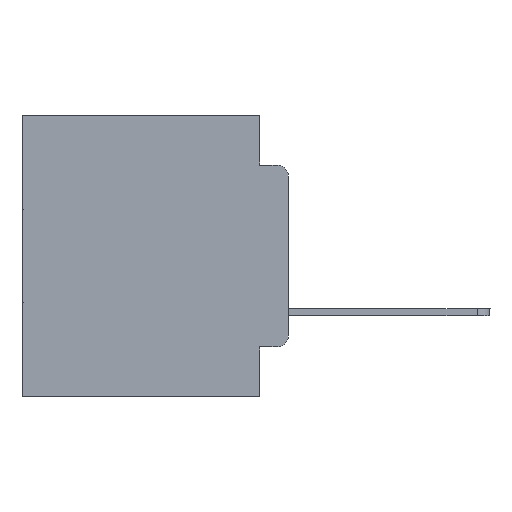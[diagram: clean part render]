
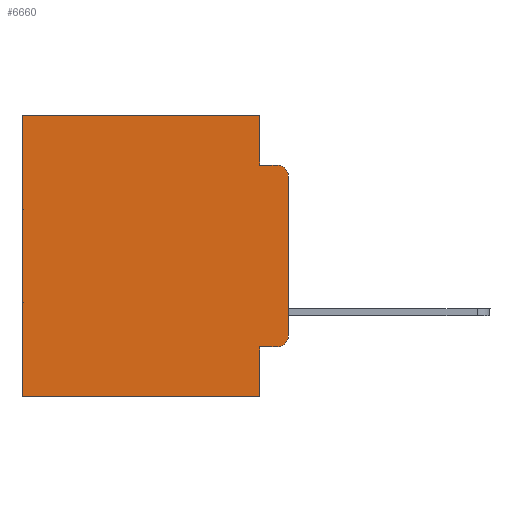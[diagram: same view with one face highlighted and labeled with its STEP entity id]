
A CAD part, left-side view. The second image highlights one B-rep face of the part: STEP entity #6660.
In plain terms, the highlighted planar face has unit normal (-1, 0, 0).
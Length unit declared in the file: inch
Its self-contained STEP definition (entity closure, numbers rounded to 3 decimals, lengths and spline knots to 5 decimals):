
#8 = AXIS2_PLACEMENT_3D ( 'NONE', #11563, #26883, #159 ) ;
#159 = DIRECTION ( 'NONE',  ( 0., 0., -1. ) ) ;
#679 = VERTEX_POINT ( 'NONE', #10246 ) ;
#705 = DIRECTION ( 'NONE',  ( 1., 0., 0. ) ) ;
#1409 = CARTESIAN_POINT ( 'NONE',  ( 0.298, 0., -0.5 ) ) ;
#1889 = CARTESIAN_POINT ( 'NONE',  ( 0.298, 0., -0.3915 ) ) ;
#2319 = LINE ( 'NONE', #21150, #7249 ) ;
#2507 = EDGE_CURVE ( 'NONE', #12230, #25333, #15939, .T. ) ;
#2879 = LINE ( 'NONE', #22156, #26074 ) ;
#4026 = VECTOR ( 'NONE', #7804, 39.37008 ) ;
#4188 = ORIENTED_EDGE ( 'NONE', *, *, #16182, .T. ) ;
#4217 = CARTESIAN_POINT ( 'NONE',  ( 0.298, 0.473, 0. ) ) ;
#4459 = ORIENTED_EDGE ( 'NONE', *, *, #10893, .T. ) ;
#4500 = LINE ( 'NONE', #9744, #17186 ) ;
#4859 = PLANE ( 'NONE',  #19401 ) ;
#4991 = VECTOR ( 'NONE', #23634, 39.37008 ) ;
#5148 = VERTEX_POINT ( 'NONE', #12575 ) ;
#5451 = CARTESIAN_POINT ( 'NONE',  ( 0.298, 0.051, -0.4115 ) ) ;
#5546 = EDGE_CURVE ( 'NONE', #8110, #5148, #10826, .T. ) ;
#5676 = EDGE_CURVE ( 'NONE', #8110, #9055, #4500, .T. ) ;
#6211 = CARTESIAN_POINT ( 'NONE',  ( 0.298, 0.051, 0. ) ) ;
#6660 = ADVANCED_FACE ( 'NONE', ( #22684 ), #4859, .F. ) ;
#7194 = LINE ( 'NONE', #17104, #4026 ) ;
#7249 = VECTOR ( 'NONE', #12591, 39.37008 ) ;
#7804 = DIRECTION ( 'NONE',  ( 0., 0., -1. ) ) ;
#8110 = VERTEX_POINT ( 'NONE', #15706 ) ;
#8390 = EDGE_CURVE ( 'NONE', #17276, #5148, #2879, .T. ) ;
#8548 = ORIENTED_EDGE ( 'NONE', *, *, #24456, .F. ) ;
#9055 = VERTEX_POINT ( 'NONE', #1889 ) ;
#9395 = VECTOR ( 'NONE', #19879, 39.37008 ) ;
#9641 = VERTEX_POINT ( 'NONE', #13053 ) ;
#9744 = CARTESIAN_POINT ( 'NONE',  ( 0.298, 0., 0. ) ) ;
#9766 = EDGE_LOOP ( 'NONE', ( #18115, #16233, #18777, #8548, #25624, #4459, #13701, #28187, #17863, #4188 ) ) ;
#10246 = CARTESIAN_POINT ( 'NONE',  ( 0.298, 0.051, 0. ) ) ;
#10755 = EDGE_CURVE ( 'NONE', #13530, #12230, #14354, .T. ) ;
#10757 = CARTESIAN_POINT ( 'NONE',  ( 0.298, 0.473, 0. ) ) ;
#10826 = CIRCLE ( 'NONE', #18111, 0.02 ) ;
#10893 = EDGE_CURVE ( 'NONE', #21752, #25333, #17518, .T. ) ;
#11563 = CARTESIAN_POINT ( 'NONE',  ( 0.298, 0.02, -0.3915 ) ) ;
#11644 = CARTESIAN_POINT ( 'NONE',  ( 0.298, 0., 0. ) ) ;
#11649 = CARTESIAN_POINT ( 'NONE',  ( 0.298, 0.02, -0.1085 ) ) ;
#12230 = VERTEX_POINT ( 'NONE', #12235 ) ;
#12235 = CARTESIAN_POINT ( 'NONE',  ( 0.298, 0.051, -0.5 ) ) ;
#12365 = DIRECTION ( 'NONE',  ( 0., 0., -1. ) ) ;
#12575 = CARTESIAN_POINT ( 'NONE',  ( 0.298, 0.02, -0.0885 ) ) ;
#12591 = DIRECTION ( 'NONE',  ( 0., 1., 0. ) ) ;
#12798 = CARTESIAN_POINT ( 'NONE',  ( 0.298, 0.051, -0.0885 ) ) ;
#13053 = CARTESIAN_POINT ( 'NONE',  ( 0.298, 0.02, -0.4115 ) ) ;
#13530 = VERTEX_POINT ( 'NONE', #5451 ) ;
#13701 = ORIENTED_EDGE ( 'NONE', *, *, #2507, .F. ) ;
#14193 = DIRECTION ( 'NONE',  ( 0., 0., -1. ) ) ;
#14354 = LINE ( 'NONE', #6211, #28741 ) ;
#15197 = CIRCLE ( 'NONE', #8, 0.02 ) ;
#15706 = CARTESIAN_POINT ( 'NONE',  ( 0.298, 0., -0.1085 ) ) ;
#15939 = LINE ( 'NONE', #1409, #27141 ) ;
#16182 = EDGE_CURVE ( 'NONE', #9641, #9055, #15197, .T. ) ;
#16233 = ORIENTED_EDGE ( 'NONE', *, *, #5546, .T. ) ;
#16902 = CARTESIAN_POINT ( 'NONE',  ( 0.298, 0.051, -0.4115 ) ) ;
#17104 = CARTESIAN_POINT ( 'NONE',  ( 0.298, 0.051, 0. ) ) ;
#17186 = VECTOR ( 'NONE', #18972, 39.37008 ) ;
#17276 = VERTEX_POINT ( 'NONE', #12798 ) ;
#17518 = LINE ( 'NONE', #10757, #9395 ) ;
#17863 = ORIENTED_EDGE ( 'NONE', *, *, #28133, .T. ) ;
#18111 = AXIS2_PLACEMENT_3D ( 'NONE', #11649, #20647, #22898 ) ;
#18115 = ORIENTED_EDGE ( 'NONE', *, *, #5676, .F. ) ;
#18777 = ORIENTED_EDGE ( 'NONE', *, *, #8390, .F. ) ;
#18972 = DIRECTION ( 'NONE',  ( 0., 0., -1. ) ) ;
#19401 = AXIS2_PLACEMENT_3D ( 'NONE', #11644, #705, #14193 ) ;
#19879 = DIRECTION ( 'NONE',  ( 0., 0., -1. ) ) ;
#20647 = DIRECTION ( 'NONE',  ( -1., 0., 0. ) ) ;
#21150 = CARTESIAN_POINT ( 'NONE',  ( 0.298, 0., 0. ) ) ;
#21752 = VERTEX_POINT ( 'NONE', #4217 ) ;
#21952 = DIRECTION ( 'NONE',  ( 0., -1., 0. ) ) ;
#22156 = CARTESIAN_POINT ( 'NONE',  ( 0.298, 0.051, -0.0885 ) ) ;
#22684 = FACE_OUTER_BOUND ( 'NONE', #9766, .T. ) ;
#22898 = DIRECTION ( 'NONE',  ( 0., 0., -1. ) ) ;
#23505 = DIRECTION ( 'NONE',  ( 0., 1., 0. ) ) ;
#23634 = DIRECTION ( 'NONE',  ( 0., -1., 0. ) ) ;
#24045 = EDGE_CURVE ( 'NONE', #679, #21752, #2319, .T. ) ;
#24159 = CARTESIAN_POINT ( 'NONE',  ( 0.298, 0.473, -0.5 ) ) ;
#24456 = EDGE_CURVE ( 'NONE', #679, #17276, #7194, .T. ) ;
#25333 = VERTEX_POINT ( 'NONE', #24159 ) ;
#25624 = ORIENTED_EDGE ( 'NONE', *, *, #24045, .T. ) ;
#26074 = VECTOR ( 'NONE', #21952, 39.37008 ) ;
#26883 = DIRECTION ( 'NONE',  ( -1., 0., 0. ) ) ;
#27120 = LINE ( 'NONE', #16902, #4991 ) ;
#27141 = VECTOR ( 'NONE', #23505, 39.37008 ) ;
#28133 = EDGE_CURVE ( 'NONE', #13530, #9641, #27120, .T. ) ;
#28187 = ORIENTED_EDGE ( 'NONE', *, *, #10755, .F. ) ;
#28741 = VECTOR ( 'NONE', #12365, 39.37008 ) ;
